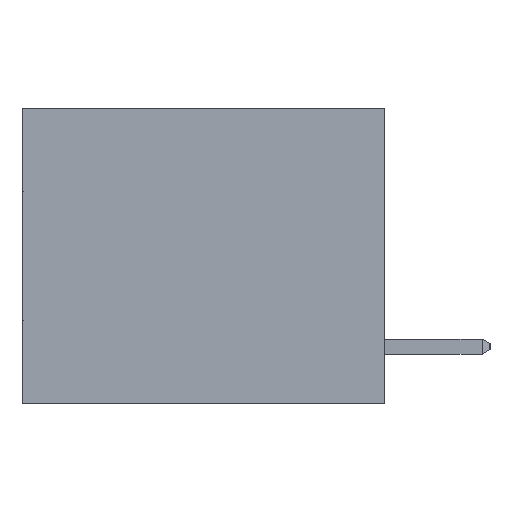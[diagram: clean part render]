
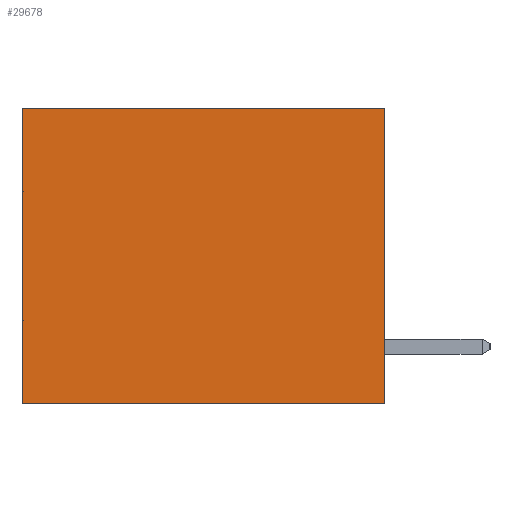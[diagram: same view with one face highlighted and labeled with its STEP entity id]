
A CAD part, left-side view. The second image highlights one B-rep face of the part: STEP entity #29678.
In plain terms, the highlighted planar face has unit normal (-1, 0, 0).
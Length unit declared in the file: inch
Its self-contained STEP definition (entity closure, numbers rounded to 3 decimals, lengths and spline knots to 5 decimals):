
#33 = DIRECTION ( 'NONE',  ( 0., 1., 0. ) ) ;
#648 = DIRECTION ( 'NONE',  ( 0., 0., -1. ) ) ;
#1550 = CARTESIAN_POINT ( 'NONE',  ( 0.3165, 0., 0. ) ) ;
#3014 = LINE ( 'NONE', #7603, #12441 ) ;
#3078 = VERTEX_POINT ( 'NONE', #22375 ) ;
#3600 = LINE ( 'NONE', #21592, #11433 ) ;
#6392 = ORIENTED_EDGE ( 'NONE', *, *, #7606, .T. ) ;
#6944 = ORIENTED_EDGE ( 'NONE', *, *, #8081, .F. ) ;
#7603 = CARTESIAN_POINT ( 'NONE',  ( 0.3165, 0., -0.49 ) ) ;
#7606 = EDGE_CURVE ( 'NONE', #31917, #18168, #10150, .T. ) ;
#8081 = EDGE_CURVE ( 'NONE', #10502, #3078, #3014, .T. ) ;
#9099 = PLANE ( 'NONE',  #23573 ) ;
#10150 = LINE ( 'NONE', #13332, #19582 ) ;
#10502 = VERTEX_POINT ( 'NONE', #24399 ) ;
#11433 = VECTOR ( 'NONE', #13821, 39.37008 ) ;
#11473 = CARTESIAN_POINT ( 'NONE',  ( 0.3165, 0., -0.49 ) ) ;
#12441 = VECTOR ( 'NONE', #33, 39.37008 ) ;
#13202 = CARTESIAN_POINT ( 'NONE',  ( 0.3165, 0., -0.49 ) ) ;
#13332 = CARTESIAN_POINT ( 'NONE',  ( 0.3165, 0., 0. ) ) ;
#13821 = DIRECTION ( 'NONE',  ( 0., 0., -1. ) ) ;
#14200 = EDGE_CURVE ( 'NONE', #18168, #3078, #3600, .T. ) ;
#18168 = VERTEX_POINT ( 'NONE', #26990 ) ;
#19582 = VECTOR ( 'NONE', #20480, 39.37008 ) ;
#20480 = DIRECTION ( 'NONE',  ( 0., 1., 0. ) ) ;
#21592 = CARTESIAN_POINT ( 'NONE',  ( 0.3165, 0.6, -0.49 ) ) ;
#22375 = CARTESIAN_POINT ( 'NONE',  ( 0.3165, 0.6, -0.49 ) ) ;
#23573 = AXIS2_PLACEMENT_3D ( 'NONE', #11473, #26352, #29159 ) ;
#24399 = CARTESIAN_POINT ( 'NONE',  ( 0.3165, 0., -0.49 ) ) ;
#25868 = VECTOR ( 'NONE', #648, 39.37008 ) ;
#25999 = EDGE_LOOP ( 'NONE', ( #27507, #6944, #30074, #6392 ) ) ;
#26352 = DIRECTION ( 'NONE',  ( 1., 0., 0. ) ) ;
#26990 = CARTESIAN_POINT ( 'NONE',  ( 0.3165, 0.6, 0. ) ) ;
#27058 = LINE ( 'NONE', #13202, #25868 ) ;
#27507 = ORIENTED_EDGE ( 'NONE', *, *, #14200, .T. ) ;
#29114 = EDGE_CURVE ( 'NONE', #31917, #10502, #27058, .T. ) ;
#29159 = DIRECTION ( 'NONE',  ( 0., 0., -1. ) ) ;
#29678 = ADVANCED_FACE ( 'NONE', ( #32557 ), #9099, .F. ) ;
#30074 = ORIENTED_EDGE ( 'NONE', *, *, #29114, .F. ) ;
#31917 = VERTEX_POINT ( 'NONE', #1550 ) ;
#32557 = FACE_OUTER_BOUND ( 'NONE', #25999, .T. ) ;
